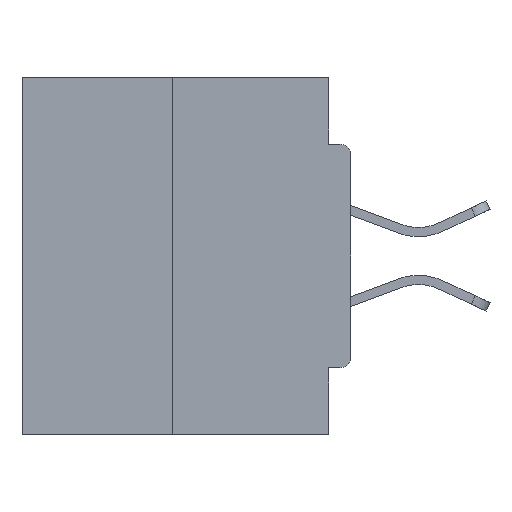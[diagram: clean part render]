
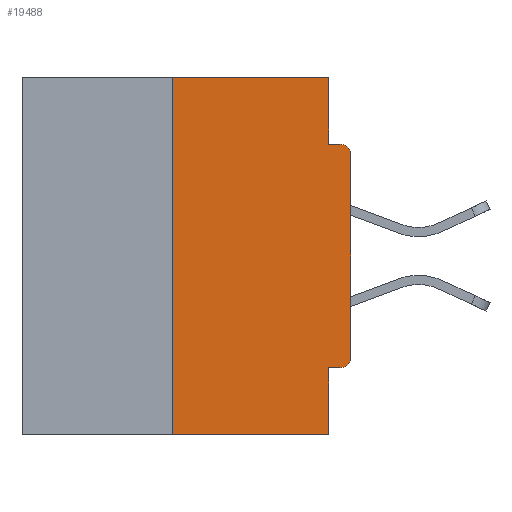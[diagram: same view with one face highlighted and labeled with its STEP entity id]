
A CAD part, left-side view. The second image highlights one B-rep face of the part: STEP entity #19488.
In plain terms, the highlighted planar face has unit normal (-1, 0, 0).
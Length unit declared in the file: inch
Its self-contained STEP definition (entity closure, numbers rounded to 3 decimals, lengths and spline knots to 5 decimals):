
#249 = DIRECTION ( 'NONE',  ( 0., 0., -1. ) ) ;
#1255 = ORIENTED_EDGE ( 'NONE', *, *, #14014, .T. ) ;
#2604 = DIRECTION ( 'NONE',  ( 0., 1., 0. ) ) ;
#2641 = DIRECTION ( 'NONE',  ( 0., 0., 1. ) ) ;
#2947 = ORIENTED_EDGE ( 'NONE', *, *, #8511, .T. ) ;
#3337 = DIRECTION ( 'NONE',  ( 0., 0., 1. ) ) ;
#3354 = DIRECTION ( 'NONE',  ( 0., 0., -1. ) ) ;
#3531 = CARTESIAN_POINT ( 'NONE',  ( 0., 0.031, 0. ) ) ;
#3559 = LINE ( 'NONE', #32782, #25954 ) ;
#3654 = DIRECTION ( 'NONE',  ( -1., 0., 0. ) ) ;
#4696 = CARTESIAN_POINT ( 'NONE',  ( 0., 0.031, -0.4065 ) ) ;
#4749 = ORIENTED_EDGE ( 'NONE', *, *, #6660, .T. ) ;
#5136 = EDGE_CURVE ( 'NONE', #32548, #16240, #10229, .T. ) ;
#5230 = LINE ( 'NONE', #15882, #7636 ) ;
#5682 = DIRECTION ( 'NONE',  ( 0., -1., 0. ) ) ;
#5991 = LINE ( 'NONE', #3531, #26887 ) ;
#6055 = EDGE_CURVE ( 'NONE', #34497, #23016, #5230, .T. ) ;
#6660 = EDGE_CURVE ( 'NONE', #34497, #8873, #23759, .T. ) ;
#6666 = FACE_OUTER_BOUND ( 'NONE', #24540, .T. ) ;
#7636 = VECTOR ( 'NONE', #2604, 39.37008 ) ;
#7860 = ORIENTED_EDGE ( 'NONE', *, *, #31742, .T. ) ;
#8435 = CARTESIAN_POINT ( 'NONE',  ( 0., 0.015, -0.1085 ) ) ;
#8511 = EDGE_CURVE ( 'NONE', #30970, #12100, #33899, .T. ) ;
#8873 = VERTEX_POINT ( 'NONE', #13146 ) ;
#9032 = ORIENTED_EDGE ( 'NONE', *, *, #5136, .F. ) ;
#9903 = CARTESIAN_POINT ( 'NONE',  ( 0., 0.015, -0.0935 ) ) ;
#10229 = LINE ( 'NONE', #20919, #23874 ) ;
#11213 = VECTOR ( 'NONE', #31098, 39.37008 ) ;
#12100 = VERTEX_POINT ( 'NONE', #12277 ) ;
#12277 = CARTESIAN_POINT ( 'NONE',  ( 0., 0.031, -0.5 ) ) ;
#12297 = CARTESIAN_POINT ( 'NONE',  ( 0., 0.015, -0.4065 ) ) ;
#13146 = CARTESIAN_POINT ( 'NONE',  ( 0., 0., -0.3915 ) ) ;
#13634 = CARTESIAN_POINT ( 'NONE',  ( 0., 0., 0. ) ) ;
#13649 = CARTESIAN_POINT ( 'NONE',  ( 0., 0.25, 0. ) ) ;
#14014 = EDGE_CURVE ( 'NONE', #8873, #28608, #15917, .T. ) ;
#14912 = CARTESIAN_POINT ( 'NONE',  ( 0., 0.25, 0. ) ) ;
#15685 = ORIENTED_EDGE ( 'NONE', *, *, #25683, .F. ) ;
#15882 = CARTESIAN_POINT ( 'NONE',  ( 0., 0., -0.4065 ) ) ;
#15917 = LINE ( 'NONE', #13634, #25592 ) ;
#16030 = ORIENTED_EDGE ( 'NONE', *, *, #32286, .F. ) ;
#16240 = VERTEX_POINT ( 'NONE', #25664 ) ;
#16342 = EDGE_CURVE ( 'NONE', #23016, #12100, #29490, .T. ) ;
#18507 = VECTOR ( 'NONE', #3337, 39.37008 ) ;
#18569 = ORIENTED_EDGE ( 'NONE', *, *, #26111, .F. ) ;
#19185 = VERTEX_POINT ( 'NONE', #30715 ) ;
#19426 = LINE ( 'NONE', #13649, #18507 ) ;
#19488 = ADVANCED_FACE ( 'NONE', ( #6666 ), #22564, .F. ) ;
#20919 = CARTESIAN_POINT ( 'NONE',  ( 0., 0.46, 0. ) ) ;
#22564 = PLANE ( 'NONE',  #22678 ) ;
#22678 = AXIS2_PLACEMENT_3D ( 'NONE', #32903, #33069, #3354 ) ;
#23000 = CARTESIAN_POINT ( 'NONE',  ( 0., 0.25, -0.5 ) ) ;
#23016 = VERTEX_POINT ( 'NONE', #4696 ) ;
#23759 = CIRCLE ( 'NONE', #33808, 0.015 ) ;
#23874 = VECTOR ( 'NONE', #30896, 39.37008 ) ;
#24540 = EDGE_LOOP ( 'NONE', ( #9032, #18569, #2947, #25401, #25089, #4749, #1255, #7860, #16030, #15685 ) ) ;
#25089 = ORIENTED_EDGE ( 'NONE', *, *, #6055, .F. ) ;
#25401 = ORIENTED_EDGE ( 'NONE', *, *, #16342, .F. ) ;
#25592 = VECTOR ( 'NONE', #2641, 39.37008 ) ;
#25664 = CARTESIAN_POINT ( 'NONE',  ( 0., 0.031, 0. ) ) ;
#25683 = EDGE_CURVE ( 'NONE', #16240, #19185, #5991, .T. ) ;
#25954 = VECTOR ( 'NONE', #5682, 39.37008 ) ;
#26111 = EDGE_CURVE ( 'NONE', #30970, #32548, #19426, .T. ) ;
#26649 = DIRECTION ( 'NONE',  ( -1., 0., 0. ) ) ;
#26871 = CARTESIAN_POINT ( 'NONE',  ( 0., 0.031, -0.5 ) ) ;
#26887 = VECTOR ( 'NONE', #32573, 39.37008 ) ;
#27156 = DIRECTION ( 'NONE',  ( 0., 0., -1. ) ) ;
#27618 = CARTESIAN_POINT ( 'NONE',  ( 0., 0.015, -0.3915 ) ) ;
#28044 = VERTEX_POINT ( 'NONE', #9903 ) ;
#28608 = VERTEX_POINT ( 'NONE', #29111 ) ;
#29111 = CARTESIAN_POINT ( 'NONE',  ( 0., 0., -0.1085 ) ) ;
#29490 = LINE ( 'NONE', #26871, #31512 ) ;
#30715 = CARTESIAN_POINT ( 'NONE',  ( 0., 0.031, -0.0935 ) ) ;
#30775 = DIRECTION ( 'NONE',  ( 0., 0., -1. ) ) ;
#30896 = DIRECTION ( 'NONE',  ( 0., -1., 0. ) ) ;
#30970 = VERTEX_POINT ( 'NONE', #23000 ) ;
#31098 = DIRECTION ( 'NONE',  ( 0., -1., 0. ) ) ;
#31512 = VECTOR ( 'NONE', #249, 39.37008 ) ;
#31742 = EDGE_CURVE ( 'NONE', #28608, #28044, #32641, .T. ) ;
#32286 = EDGE_CURVE ( 'NONE', #19185, #28044, #3559, .T. ) ;
#32548 = VERTEX_POINT ( 'NONE', #14912 ) ;
#32573 = DIRECTION ( 'NONE',  ( 0., 0., -1. ) ) ;
#32641 = CIRCLE ( 'NONE', #33178, 0.015 ) ;
#32782 = CARTESIAN_POINT ( 'NONE',  ( 0., 0., -0.0935 ) ) ;
#32903 = CARTESIAN_POINT ( 'NONE',  ( 0., 0.46, 0. ) ) ;
#33069 = DIRECTION ( 'NONE',  ( 1., 0., 0. ) ) ;
#33178 = AXIS2_PLACEMENT_3D ( 'NONE', #8435, #26649, #27156 ) ;
#33386 = CARTESIAN_POINT ( 'NONE',  ( 0., 0.46, -0.5 ) ) ;
#33808 = AXIS2_PLACEMENT_3D ( 'NONE', #27618, #3654, #30775 ) ;
#33899 = LINE ( 'NONE', #33386, #11213 ) ;
#34497 = VERTEX_POINT ( 'NONE', #12297 ) ;
